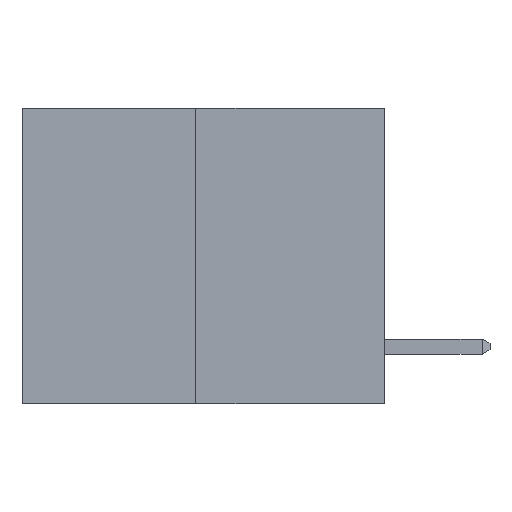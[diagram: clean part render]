
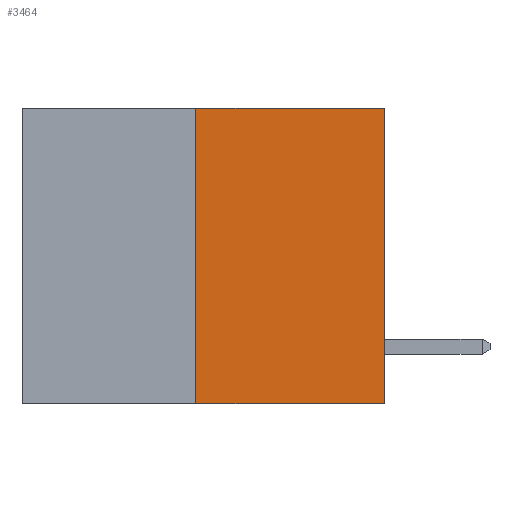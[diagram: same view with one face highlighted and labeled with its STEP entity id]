
A CAD part, left-side view. The second image highlights one B-rep face of the part: STEP entity #3464.
In plain terms, the highlighted planar face has unit normal (-1, 0, 0).
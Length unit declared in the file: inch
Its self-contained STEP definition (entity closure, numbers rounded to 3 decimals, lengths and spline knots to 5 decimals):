
#314 = DIRECTION ( 'NONE',  ( 1., 0., 0. ) ) ;
#531 = VERTEX_POINT ( 'NONE', #3221 ) ;
#621 = VECTOR ( 'NONE', #3848, 39.37008 ) ;
#741 = ORIENTED_EDGE ( 'NONE', *, *, #3107, .T. ) ;
#752 = EDGE_CURVE ( 'NONE', #531, #8510, #6194, .T. ) ;
#2122 = DIRECTION ( 'NONE',  ( 0., 0., 1. ) ) ;
#2378 = DIRECTION ( 'NONE',  ( 0., -1., 0. ) ) ;
#2412 = DIRECTION ( 'NONE',  ( 0., 0., -1. ) ) ;
#2953 = EDGE_CURVE ( 'NONE', #3530, #5709, #8585, .T. ) ;
#3086 = ORIENTED_EDGE ( 'NONE', *, *, #2953, .T. ) ;
#3107 = EDGE_CURVE ( 'NONE', #531, #3530, #3240, .T. ) ;
#3221 = CARTESIAN_POINT ( 'NONE',  ( 0., 0.312, -0.49 ) ) ;
#3240 = LINE ( 'NONE', #4053, #3680 ) ;
#3464 = ADVANCED_FACE ( 'NONE', ( #6610 ), #3573, .F. ) ;
#3530 = VERTEX_POINT ( 'NONE', #5761 ) ;
#3573 = PLANE ( 'NONE',  #8059 ) ;
#3599 = CARTESIAN_POINT ( 'NONE',  ( 0., 0.6, 0. ) ) ;
#3680 = VECTOR ( 'NONE', #6088, 39.37008 ) ;
#3848 = DIRECTION ( 'NONE',  ( 0., 0., 1. ) ) ;
#3850 = CARTESIAN_POINT ( 'NONE',  ( 0., 0., 0. ) ) ;
#4053 = CARTESIAN_POINT ( 'NONE',  ( 0., 0.6, -0.49 ) ) ;
#4403 = EDGE_CURVE ( 'NONE', #8510, #5709, #5616, .T. ) ;
#4771 = VECTOR ( 'NONE', #2122, 39.37008 ) ;
#5377 = VECTOR ( 'NONE', #2378, 39.37008 ) ;
#5550 = CARTESIAN_POINT ( 'NONE',  ( 0., 0.312, -0.49 ) ) ;
#5616 = LINE ( 'NONE', #6508, #5377 ) ;
#5684 = EDGE_LOOP ( 'NONE', ( #6953, #741, #3086, #8779 ) ) ;
#5709 = VERTEX_POINT ( 'NONE', #3850 ) ;
#5761 = CARTESIAN_POINT ( 'NONE',  ( 0., 0., -0.49 ) ) ;
#6088 = DIRECTION ( 'NONE',  ( 0., -1., 0. ) ) ;
#6194 = LINE ( 'NONE', #5550, #4771 ) ;
#6508 = CARTESIAN_POINT ( 'NONE',  ( 0., 0.6, 0. ) ) ;
#6604 = CARTESIAN_POINT ( 'NONE',  ( 0., 0.312, 0. ) ) ;
#6610 = FACE_OUTER_BOUND ( 'NONE', #5684, .T. ) ;
#6953 = ORIENTED_EDGE ( 'NONE', *, *, #752, .F. ) ;
#7049 = CARTESIAN_POINT ( 'NONE',  ( 0., 0., 0. ) ) ;
#8059 = AXIS2_PLACEMENT_3D ( 'NONE', #3599, #314, #2412 ) ;
#8510 = VERTEX_POINT ( 'NONE', #6604 ) ;
#8585 = LINE ( 'NONE', #7049, #621 ) ;
#8779 = ORIENTED_EDGE ( 'NONE', *, *, #4403, .F. ) ;
